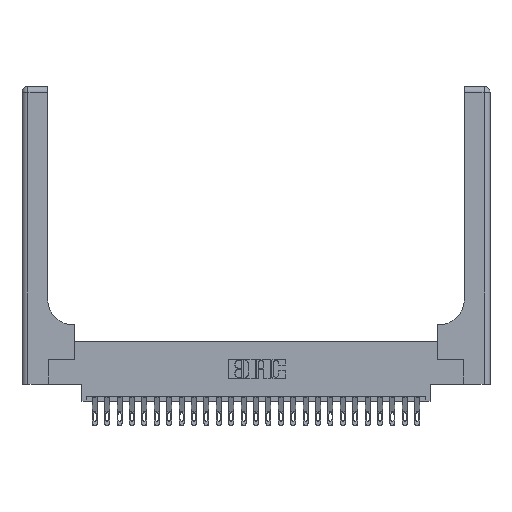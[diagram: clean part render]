
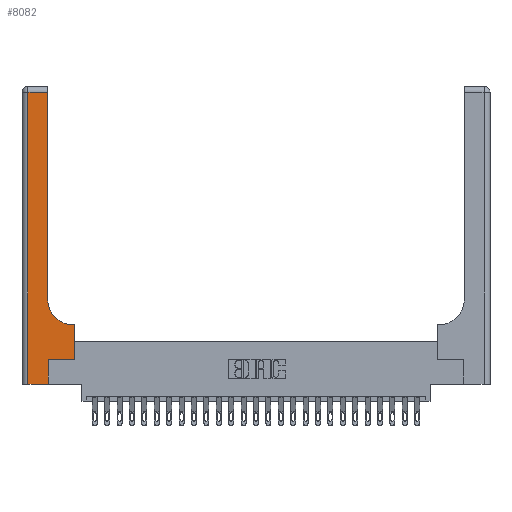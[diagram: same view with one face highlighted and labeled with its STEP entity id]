
A CAD part, top view. The second image highlights one B-rep face of the part: STEP entity #8082.
In plain terms, the highlighted planar face has unit normal (0, 0, 1).
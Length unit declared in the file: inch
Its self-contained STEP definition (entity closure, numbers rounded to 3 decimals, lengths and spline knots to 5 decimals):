
#95 = VERTEX_POINT ( 'NONE', #9658 ) ;
#148 = CARTESIAN_POINT ( 'NONE',  ( 0.06, 0., 0.37 ) ) ;
#584 = CARTESIAN_POINT ( 'NONE',  ( 0.528, 0.25, 0.37 ) ) ;
#1214 = DIRECTION ( 'NONE',  ( -1., 0., 0. ) ) ;
#1364 = CIRCLE ( 'NONE', #11354, 0.25 ) ;
#1778 = VECTOR ( 'NONE', #23661, 39.37008 ) ;
#1891 = DIRECTION ( 'NONE',  ( 0., 1., 0. ) ) ;
#2766 = CARTESIAN_POINT ( 'NONE',  ( 0.26, 0.85, 0.37 ) ) ;
#2798 = CARTESIAN_POINT ( 'NONE',  ( 0.26, 2.94, 0.37 ) ) ;
#2943 = LINE ( 'NONE', #8547, #4916 ) ;
#3207 = LINE ( 'NONE', #13113, #16788 ) ;
#3476 = DIRECTION ( 'NONE',  ( 0., -1., 0. ) ) ;
#3908 = ORIENTED_EDGE ( 'NONE', *, *, #11048, .T. ) ;
#4082 = EDGE_CURVE ( 'NONE', #10086, #21204, #24661, .T. ) ;
#4420 = VECTOR ( 'NONE', #1214, 39.37008 ) ;
#4524 = DIRECTION ( 'NONE',  ( 1., 0., 0. ) ) ;
#4916 = VECTOR ( 'NONE', #24689, 39.37008 ) ;
#5290 = DIRECTION ( 'NONE',  ( 1., 0., 0. ) ) ;
#5404 = VERTEX_POINT ( 'NONE', #11500 ) ;
#7551 = ORIENTED_EDGE ( 'NONE', *, *, #12329, .T. ) ;
#7648 = VECTOR ( 'NONE', #3476, 39.37008 ) ;
#8082 = ADVANCED_FACE ( 'NONE', ( #18852 ), #11032, .F. ) ;
#8547 = CARTESIAN_POINT ( 'NONE',  ( 0.26, 0.6, 0.37 ) ) ;
#9116 = DIRECTION ( 'NONE',  ( 1., 0., 0. ) ) ;
#9221 = EDGE_LOOP ( 'NONE', ( #25475, #11078, #23538, #12237, #3908, #7551, #16706, #17900, #17225 ) ) ;
#9658 = CARTESIAN_POINT ( 'NONE',  ( 0.265, 0., 0.37 ) ) ;
#10086 = VERTEX_POINT ( 'NONE', #2798 ) ;
#10188 = AXIS2_PLACEMENT_3D ( 'NONE', #10903, #25228, #20929 ) ;
#10438 = VERTEX_POINT ( 'NONE', #2766 ) ;
#10653 = LINE ( 'NONE', #24076, #14153 ) ;
#10796 = VERTEX_POINT ( 'NONE', #148 ) ;
#10903 = CARTESIAN_POINT ( 'NONE',  ( 0., 3., 0.37 ) ) ;
#11032 = PLANE ( 'NONE',  #10188 ) ;
#11048 = EDGE_CURVE ( 'NONE', #95, #15953, #17302, .T. ) ;
#11078 = ORIENTED_EDGE ( 'NONE', *, *, #4082, .T. ) ;
#11354 = AXIS2_PLACEMENT_3D ( 'NONE', #16804, #16544, #9116 ) ;
#11500 = CARTESIAN_POINT ( 'NONE',  ( 0.51, 0.6, 0.37 ) ) ;
#12237 = ORIENTED_EDGE ( 'NONE', *, *, #18506, .T. ) ;
#12329 = EDGE_CURVE ( 'NONE', #15953, #17515, #10653, .T. ) ;
#12499 = CARTESIAN_POINT ( 'NONE',  ( 0.26, 3., 0.37 ) ) ;
#13113 = CARTESIAN_POINT ( 'NONE',  ( 0., 0., 0.37 ) ) ;
#13197 = CARTESIAN_POINT ( 'NONE',  ( 0., 2.94, 0.37 ) ) ;
#14153 = VECTOR ( 'NONE', #4524, 39.37008 ) ;
#14857 = VECTOR ( 'NONE', #1891, 39.37008 ) ;
#14925 = EDGE_CURVE ( 'NONE', #10438, #10086, #23267, .T. ) ;
#15872 = EDGE_CURVE ( 'NONE', #5404, #10438, #1364, .T. ) ;
#15953 = VERTEX_POINT ( 'NONE', #20711 ) ;
#16544 = DIRECTION ( 'NONE',  ( 0., 0., -1. ) ) ;
#16706 = ORIENTED_EDGE ( 'NONE', *, *, #22603, .T. ) ;
#16788 = VECTOR ( 'NONE', #5290, 39.37008 ) ;
#16804 = CARTESIAN_POINT ( 'NONE',  ( 0.51, 0.85, 0.37 ) ) ;
#17042 = CARTESIAN_POINT ( 'NONE',  ( 0.265, 0., 0.37 ) ) ;
#17225 = ORIENTED_EDGE ( 'NONE', *, *, #15872, .T. ) ;
#17302 = LINE ( 'NONE', #17042, #21100 ) ;
#17515 = VERTEX_POINT ( 'NONE', #584 ) ;
#17900 = ORIENTED_EDGE ( 'NONE', *, *, #24129, .T. ) ;
#18506 = EDGE_CURVE ( 'NONE', #10796, #95, #3207, .T. ) ;
#18558 = EDGE_CURVE ( 'NONE', #21204, #10796, #21312, .T. ) ;
#18852 = FACE_OUTER_BOUND ( 'NONE', #9221, .T. ) ;
#19858 = CARTESIAN_POINT ( 'NONE',  ( 0.528, 0.25, 0.37 ) ) ;
#20213 = CARTESIAN_POINT ( 'NONE',  ( 0.528, 0.6, 0.37 ) ) ;
#20711 = CARTESIAN_POINT ( 'NONE',  ( 0.265, 0.25, 0.37 ) ) ;
#20929 = DIRECTION ( 'NONE',  ( -1., 0., 0. ) ) ;
#21100 = VECTOR ( 'NONE', #21214, 39.37008 ) ;
#21204 = VERTEX_POINT ( 'NONE', #23239 ) ;
#21214 = DIRECTION ( 'NONE',  ( 0., 1., 0. ) ) ;
#21312 = LINE ( 'NONE', #24955, #7648 ) ;
#22603 = EDGE_CURVE ( 'NONE', #17515, #25347, #23628, .T. ) ;
#23239 = CARTESIAN_POINT ( 'NONE',  ( 0.06, 2.94, 0.37 ) ) ;
#23267 = LINE ( 'NONE', #12499, #1778 ) ;
#23538 = ORIENTED_EDGE ( 'NONE', *, *, #18558, .T. ) ;
#23628 = LINE ( 'NONE', #19858, #14857 ) ;
#23661 = DIRECTION ( 'NONE',  ( 0., 1., 0. ) ) ;
#24076 = CARTESIAN_POINT ( 'NONE',  ( 0.265, 0.25, 0.37 ) ) ;
#24129 = EDGE_CURVE ( 'NONE', #25347, #5404, #2943, .T. ) ;
#24661 = LINE ( 'NONE', #13197, #4420 ) ;
#24689 = DIRECTION ( 'NONE',  ( -1., 0., 0. ) ) ;
#24955 = CARTESIAN_POINT ( 'NONE',  ( 0.06, 3., 0.37 ) ) ;
#25228 = DIRECTION ( 'NONE',  ( 0., 0., -1. ) ) ;
#25347 = VERTEX_POINT ( 'NONE', #20213 ) ;
#25475 = ORIENTED_EDGE ( 'NONE', *, *, #14925, .T. ) ;
